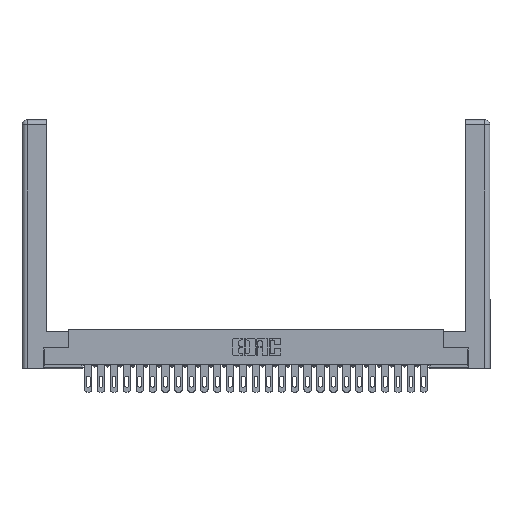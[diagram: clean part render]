
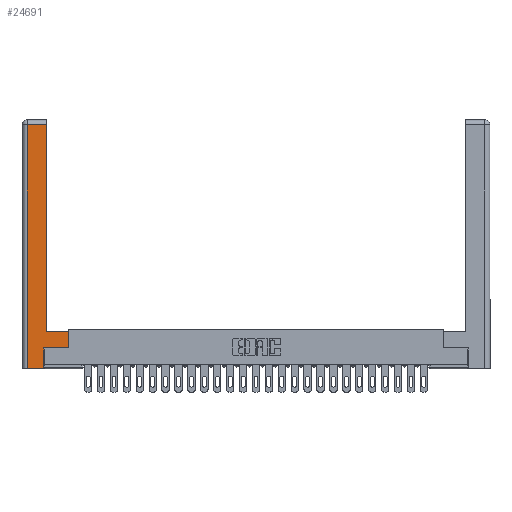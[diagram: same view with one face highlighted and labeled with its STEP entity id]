
A CAD part, top view. The second image highlights one B-rep face of the part: STEP entity #24691.
In plain terms, the highlighted planar face has unit normal (0, 0, 1).
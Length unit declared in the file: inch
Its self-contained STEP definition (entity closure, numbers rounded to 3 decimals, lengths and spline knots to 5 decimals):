
#249 = CARTESIAN_POINT ( 'NONE',  ( 0., 0., 0. ) ) ;
#413 = ORIENTED_EDGE ( 'NONE', *, *, #5164, .T. ) ;
#985 = CARTESIAN_POINT ( 'NONE',  ( 0.265, 0.245, 0. ) ) ;
#1325 = EDGE_LOOP ( 'NONE', ( #413, #11812, #17512, #5173, #7999, #8074, #20542, #5519 ) ) ;
#2225 = CARTESIAN_POINT ( 'NONE',  ( 0.0615, 2.94, 0. ) ) ;
#2397 = CARTESIAN_POINT ( 'NONE',  ( 0.565, 0.245, 0. ) ) ;
#2497 = DIRECTION ( 'NONE',  ( -1., 0., 0. ) ) ;
#2699 = DIRECTION ( 'NONE',  ( 1., 0., 0. ) ) ;
#2702 = VECTOR ( 'NONE', #18409, 39.37008 ) ;
#3248 = DIRECTION ( 'NONE',  ( 0., 1., 0. ) ) ;
#4197 = AXIS2_PLACEMENT_3D ( 'NONE', #249, #10654, #21222 ) ;
#4292 = VECTOR ( 'NONE', #3248, 39.37008 ) ;
#4515 = EDGE_CURVE ( 'NONE', #21869, #15186, #17065, .T. ) ;
#5035 = EDGE_CURVE ( 'NONE', #22329, #10096, #18368, .T. ) ;
#5164 = EDGE_CURVE ( 'NONE', #14891, #27466, #17675, .T. ) ;
#5173 = ORIENTED_EDGE ( 'NONE', *, *, #4515, .T. ) ;
#5519 = ORIENTED_EDGE ( 'NONE', *, *, #21339, .T. ) ;
#6981 = CARTESIAN_POINT ( 'NONE',  ( 0.265, 0., 0. ) ) ;
#7284 = LINE ( 'NONE', #2225, #12254 ) ;
#7320 = CARTESIAN_POINT ( 'NONE',  ( 0.565, 0.45, 0. ) ) ;
#7999 = ORIENTED_EDGE ( 'NONE', *, *, #23549, .T. ) ;
#8074 = ORIENTED_EDGE ( 'NONE', *, *, #5035, .T. ) ;
#8435 = PLANE ( 'NONE',  #4197 ) ;
#9665 = VECTOR ( 'NONE', #22184, 39.37008 ) ;
#10096 = VERTEX_POINT ( 'NONE', #14000 ) ;
#10654 = DIRECTION ( 'NONE',  ( 0., 0., -1. ) ) ;
#11171 = CARTESIAN_POINT ( 'NONE',  ( 0.295, 0.45, 0. ) ) ;
#11451 = VECTOR ( 'NONE', #2699, 39.37008 ) ;
#11812 = ORIENTED_EDGE ( 'NONE', *, *, #18948, .T. ) ;
#12254 = VECTOR ( 'NONE', #2497, 39.37008 ) ;
#12430 = CARTESIAN_POINT ( 'NONE',  ( 0.0615, 0., 0. ) ) ;
#12588 = LINE ( 'NONE', #16041, #4292 ) ;
#13233 = DIRECTION ( 'NONE',  ( 1., 0., 0. ) ) ;
#14000 = CARTESIAN_POINT ( 'NONE',  ( 0.565, 0.245, 0. ) ) ;
#14025 = LINE ( 'NONE', #11171, #2702 ) ;
#14304 = VERTEX_POINT ( 'NONE', #18810 ) ;
#14891 = VERTEX_POINT ( 'NONE', #16466 ) ;
#15186 = VERTEX_POINT ( 'NONE', #15939 ) ;
#15939 = CARTESIAN_POINT ( 'NONE',  ( 0.265, 0., 0. ) ) ;
#16041 = CARTESIAN_POINT ( 'NONE',  ( 0.265, 0.245, 0. ) ) ;
#16466 = CARTESIAN_POINT ( 'NONE',  ( 0.295, 0.45, 0. ) ) ;
#16501 = EDGE_CURVE ( 'NONE', #26018, #21869, #18363, .T. ) ;
#17065 = LINE ( 'NONE', #6981, #11451 ) ;
#17512 = ORIENTED_EDGE ( 'NONE', *, *, #16501, .T. ) ;
#17528 = CARTESIAN_POINT ( 'NONE',  ( 0.0615, 2.94, 0. ) ) ;
#17675 = LINE ( 'NONE', #20676, #18339 ) ;
#18324 = DIRECTION ( 'NONE',  ( 0., -1., 0. ) ) ;
#18339 = VECTOR ( 'NONE', #22958, 39.37008 ) ;
#18363 = LINE ( 'NONE', #20085, #26774 ) ;
#18368 = LINE ( 'NONE', #2397, #27112 ) ;
#18403 = EDGE_CURVE ( 'NONE', #10096, #14304, #20920, .T. ) ;
#18409 = DIRECTION ( 'NONE',  ( -1., 0., 0. ) ) ;
#18810 = CARTESIAN_POINT ( 'NONE',  ( 0.565, 0.45, 0. ) ) ;
#18948 = EDGE_CURVE ( 'NONE', #27466, #26018, #7284, .T. ) ;
#20085 = CARTESIAN_POINT ( 'NONE',  ( 0.0615, 0., 0. ) ) ;
#20483 = FACE_OUTER_BOUND ( 'NONE', #1325, .T. ) ;
#20542 = ORIENTED_EDGE ( 'NONE', *, *, #18403, .T. ) ;
#20676 = CARTESIAN_POINT ( 'NONE',  ( 0.295, 3., 0. ) ) ;
#20920 = LINE ( 'NONE', #7320, #9665 ) ;
#21222 = DIRECTION ( 'NONE',  ( -1., 0., 0. ) ) ;
#21339 = EDGE_CURVE ( 'NONE', #14304, #14891, #14025, .T. ) ;
#21869 = VERTEX_POINT ( 'NONE', #12430 ) ;
#22184 = DIRECTION ( 'NONE',  ( 0., 1., 0. ) ) ;
#22329 = VERTEX_POINT ( 'NONE', #985 ) ;
#22958 = DIRECTION ( 'NONE',  ( 0., 1., 0. ) ) ;
#23549 = EDGE_CURVE ( 'NONE', #15186, #22329, #12588, .T. ) ;
#24691 = ADVANCED_FACE ( 'NONE', ( #20483 ), #8435, .F. ) ;
#26018 = VERTEX_POINT ( 'NONE', #17528 ) ;
#26072 = CARTESIAN_POINT ( 'NONE',  ( 0.295, 2.94, 0. ) ) ;
#26774 = VECTOR ( 'NONE', #18324, 39.37008 ) ;
#27112 = VECTOR ( 'NONE', #13233, 39.37008 ) ;
#27466 = VERTEX_POINT ( 'NONE', #26072 ) ;
